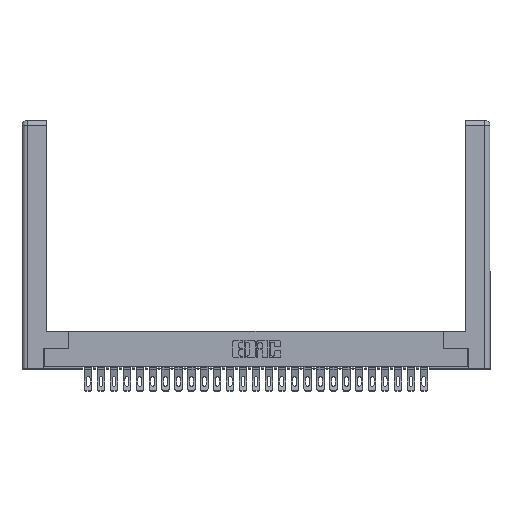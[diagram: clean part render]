
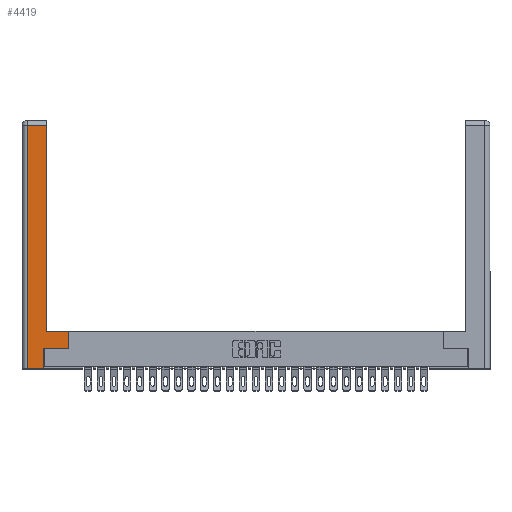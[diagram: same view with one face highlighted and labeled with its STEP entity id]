
A CAD part, top view. The second image highlights one B-rep face of the part: STEP entity #4419.
In plain terms, the highlighted planar face has unit normal (0, 0, 1).
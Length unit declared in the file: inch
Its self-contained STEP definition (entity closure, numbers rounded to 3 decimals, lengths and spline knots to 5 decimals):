
#11 = CARTESIAN_POINT ( 'NONE',  ( 0., 0., 0. ) ) ;
#451 = CARTESIAN_POINT ( 'NONE',  ( 0.0615, 0., 0. ) ) ;
#2603 = ORIENTED_EDGE ( 'NONE', *, *, #13071, .T. ) ;
#2799 = CARTESIAN_POINT ( 'NONE',  ( 0.295, 0.45, 0. ) ) ;
#2914 = DIRECTION ( 'NONE',  ( -1., 0., 0. ) ) ;
#3871 = ORIENTED_EDGE ( 'NONE', *, *, #5788, .T. ) ;
#3974 = CARTESIAN_POINT ( 'NONE',  ( 0.265, 0., 0. ) ) ;
#4140 = CARTESIAN_POINT ( 'NONE',  ( 0.0615, 0., 0. ) ) ;
#4419 = ADVANCED_FACE ( 'NONE', ( #26064 ), #18683, .F. ) ;
#4593 = EDGE_CURVE ( 'NONE', #11320, #29781, #10701, .T. ) ;
#4798 = EDGE_CURVE ( 'NONE', #28117, #21893, #7025, .T. ) ;
#5606 = CARTESIAN_POINT ( 'NONE',  ( 0.265, 0., 0. ) ) ;
#5759 = LINE ( 'NONE', #451, #20666 ) ;
#5777 = VECTOR ( 'NONE', #20751, 39.37008 ) ;
#5788 = EDGE_CURVE ( 'NONE', #13883, #11320, #18552, .T. ) ;
#5925 = ORIENTED_EDGE ( 'NONE', *, *, #4593, .T. ) ;
#6852 = VERTEX_POINT ( 'NONE', #33855 ) ;
#7025 = LINE ( 'NONE', #28695, #5777 ) ;
#7403 = VECTOR ( 'NONE', #32669, 39.37008 ) ;
#7670 = DIRECTION ( 'NONE',  ( 0., 0., -1. ) ) ;
#8638 = DIRECTION ( 'NONE',  ( 1., 0., 0. ) ) ;
#8772 = EDGE_CURVE ( 'NONE', #21893, #6852, #14931, .T. ) ;
#8971 = EDGE_CURVE ( 'NONE', #29781, #17696, #22796, .T. ) ;
#9136 = CARTESIAN_POINT ( 'NONE',  ( 0.265, 0.245, 0. ) ) ;
#10701 = LINE ( 'NONE', #9136, #7403 ) ;
#11051 = CARTESIAN_POINT ( 'NONE',  ( 0.0615, 2.94, 0. ) ) ;
#11320 = VERTEX_POINT ( 'NONE', #3974 ) ;
#12152 = CARTESIAN_POINT ( 'NONE',  ( 0.265, 0.245, 0. ) ) ;
#13071 = EDGE_CURVE ( 'NONE', #32069, #28117, #29095, .T. ) ;
#13332 = VECTOR ( 'NONE', #2914, 39.37008 ) ;
#13883 = VERTEX_POINT ( 'NONE', #4140 ) ;
#14931 = LINE ( 'NONE', #11051, #18230 ) ;
#15168 = ORIENTED_EDGE ( 'NONE', *, *, #4798, .T. ) ;
#15466 = ORIENTED_EDGE ( 'NONE', *, *, #8772, .T. ) ;
#17189 = CARTESIAN_POINT ( 'NONE',  ( 0.565, 0.45, 0. ) ) ;
#17696 = VERTEX_POINT ( 'NONE', #20386 ) ;
#17704 = CARTESIAN_POINT ( 'NONE',  ( 0.295, 2.94, 0. ) ) ;
#18230 = VECTOR ( 'NONE', #23932, 39.37008 ) ;
#18344 = EDGE_CURVE ( 'NONE', #17696, #32069, #26289, .T. ) ;
#18552 = LINE ( 'NONE', #5606, #30113 ) ;
#18683 = PLANE ( 'NONE',  #19122 ) ;
#19122 = AXIS2_PLACEMENT_3D ( 'NONE', #11, #7670, #28969 ) ;
#19887 = DIRECTION ( 'NONE',  ( 0., 1., 0. ) ) ;
#20386 = CARTESIAN_POINT ( 'NONE',  ( 0.565, 0.245, 0. ) ) ;
#20666 = VECTOR ( 'NONE', #29519, 39.37008 ) ;
#20751 = DIRECTION ( 'NONE',  ( 0., 1., 0. ) ) ;
#21696 = ORIENTED_EDGE ( 'NONE', *, *, #8971, .T. ) ;
#21893 = VERTEX_POINT ( 'NONE', #17704 ) ;
#22572 = EDGE_CURVE ( 'NONE', #6852, #13883, #5759, .T. ) ;
#22796 = LINE ( 'NONE', #24517, #27747 ) ;
#23589 = ORIENTED_EDGE ( 'NONE', *, *, #18344, .T. ) ;
#23932 = DIRECTION ( 'NONE',  ( -1., 0., 0. ) ) ;
#24517 = CARTESIAN_POINT ( 'NONE',  ( 0.565, 0.245, 0. ) ) ;
#24644 = VECTOR ( 'NONE', #19887, 39.37008 ) ;
#26064 = FACE_OUTER_BOUND ( 'NONE', #33239, .T. ) ;
#26289 = LINE ( 'NONE', #17189, #24644 ) ;
#26337 = DIRECTION ( 'NONE',  ( 1., 0., 0. ) ) ;
#26660 = CARTESIAN_POINT ( 'NONE',  ( 0.565, 0.45, 0. ) ) ;
#27747 = VECTOR ( 'NONE', #8638, 39.37008 ) ;
#28117 = VERTEX_POINT ( 'NONE', #33742 ) ;
#28695 = CARTESIAN_POINT ( 'NONE',  ( 0.295, 3., 0. ) ) ;
#28969 = DIRECTION ( 'NONE',  ( -1., 0., 0. ) ) ;
#29095 = LINE ( 'NONE', #2799, #13332 ) ;
#29519 = DIRECTION ( 'NONE',  ( 0., -1., 0. ) ) ;
#29781 = VERTEX_POINT ( 'NONE', #12152 ) ;
#30113 = VECTOR ( 'NONE', #26337, 39.37008 ) ;
#30963 = ORIENTED_EDGE ( 'NONE', *, *, #22572, .T. ) ;
#32069 = VERTEX_POINT ( 'NONE', #26660 ) ;
#32669 = DIRECTION ( 'NONE',  ( 0., 1., 0. ) ) ;
#33239 = EDGE_LOOP ( 'NONE', ( #15168, #15466, #30963, #3871, #5925, #21696, #23589, #2603 ) ) ;
#33742 = CARTESIAN_POINT ( 'NONE',  ( 0.295, 0.45, 0. ) ) ;
#33855 = CARTESIAN_POINT ( 'NONE',  ( 0.0615, 2.94, 0. ) ) ;
